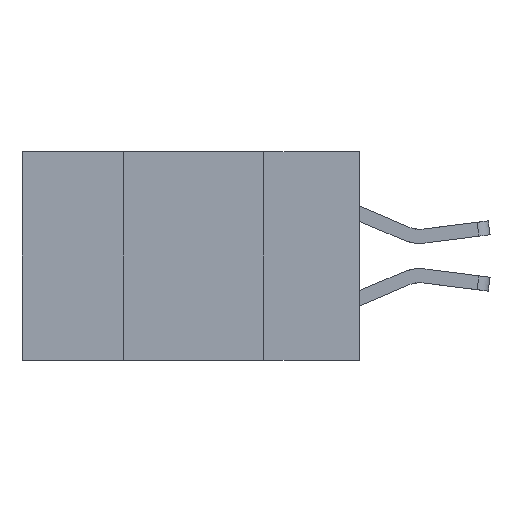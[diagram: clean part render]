
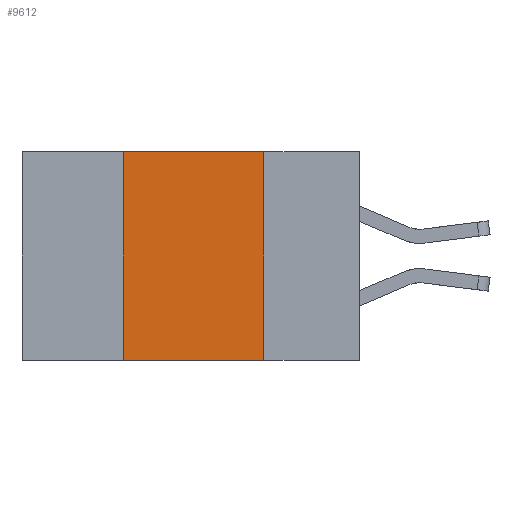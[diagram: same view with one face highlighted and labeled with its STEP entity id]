
A CAD part, left-side view. The second image highlights one B-rep face of the part: STEP entity #9612.
In plain terms, the highlighted planar face has unit normal (-1, 0, 0).
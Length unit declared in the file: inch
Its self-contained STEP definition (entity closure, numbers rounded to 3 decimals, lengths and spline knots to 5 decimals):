
#452 = VECTOR ( 'NONE', #6071, 39.37008 ) ;
#597 = DIRECTION ( 'NONE',  ( 0., 0., 1. ) ) ;
#631 = CARTESIAN_POINT ( 'NONE',  ( 0., 0.6, 0. ) ) ;
#1000 = LINE ( 'NONE', #1075, #5384 ) ;
#1075 = CARTESIAN_POINT ( 'NONE',  ( 0., 0.17, 0. ) ) ;
#1261 = LINE ( 'NONE', #6002, #5183 ) ;
#1351 = VERTEX_POINT ( 'NONE', #6048 ) ;
#1483 = EDGE_LOOP ( 'NONE', ( #9471, #2595, #6894, #2050 ) ) ;
#1611 = EDGE_CURVE ( 'NONE', #4880, #1351, #4557, .T. ) ;
#1770 = DIRECTION ( 'NONE',  ( 0., -1., 0. ) ) ;
#1862 = PLANE ( 'NONE',  #2819 ) ;
#2050 = ORIENTED_EDGE ( 'NONE', *, *, #3509, .T. ) ;
#2425 = VERTEX_POINT ( 'NONE', #9688 ) ;
#2595 = ORIENTED_EDGE ( 'NONE', *, *, #1611, .F. ) ;
#2659 = CARTESIAN_POINT ( 'NONE',  ( 0., 0.6, 0. ) ) ;
#2674 = EDGE_CURVE ( 'NONE', #1351, #4969, #1000, .T. ) ;
#2819 = AXIS2_PLACEMENT_3D ( 'NONE', #2659, #3686, #9906 ) ;
#3283 = FACE_OUTER_BOUND ( 'NONE', #1483, .T. ) ;
#3509 = EDGE_CURVE ( 'NONE', #2425, #4969, #9253, .T. ) ;
#3686 = DIRECTION ( 'NONE',  ( 1., 0., 0. ) ) ;
#4557 = LINE ( 'NONE', #631, #452 ) ;
#4656 = CARTESIAN_POINT ( 'NONE',  ( 0., 0.6, -0.37 ) ) ;
#4880 = VERTEX_POINT ( 'NONE', #8093 ) ;
#4969 = VERTEX_POINT ( 'NONE', #5868 ) ;
#5131 = VECTOR ( 'NONE', #1770, 39.37008 ) ;
#5183 = VECTOR ( 'NONE', #597, 39.37008 ) ;
#5384 = VECTOR ( 'NONE', #6397, 39.37008 ) ;
#5868 = CARTESIAN_POINT ( 'NONE',  ( 0., 0.17, -0.37 ) ) ;
#6002 = CARTESIAN_POINT ( 'NONE',  ( 0., 0.42, 0. ) ) ;
#6048 = CARTESIAN_POINT ( 'NONE',  ( 0., 0.17, 0. ) ) ;
#6071 = DIRECTION ( 'NONE',  ( 0., -1., 0. ) ) ;
#6397 = DIRECTION ( 'NONE',  ( 0., 0., -1. ) ) ;
#6894 = ORIENTED_EDGE ( 'NONE', *, *, #7753, .F. ) ;
#7753 = EDGE_CURVE ( 'NONE', #2425, #4880, #1261, .T. ) ;
#8093 = CARTESIAN_POINT ( 'NONE',  ( 0., 0.42, 0. ) ) ;
#9253 = LINE ( 'NONE', #4656, #5131 ) ;
#9471 = ORIENTED_EDGE ( 'NONE', *, *, #2674, .F. ) ;
#9612 = ADVANCED_FACE ( 'NONE', ( #3283 ), #1862, .F. ) ;
#9688 = CARTESIAN_POINT ( 'NONE',  ( 0., 0.42, -0.37 ) ) ;
#9906 = DIRECTION ( 'NONE',  ( 0., 0., -1. ) ) ;
